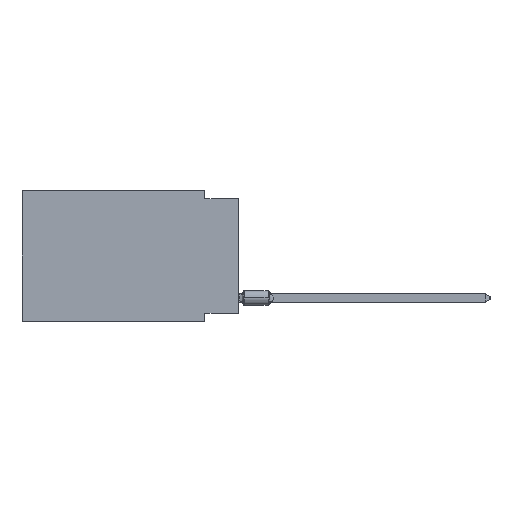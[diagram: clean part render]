
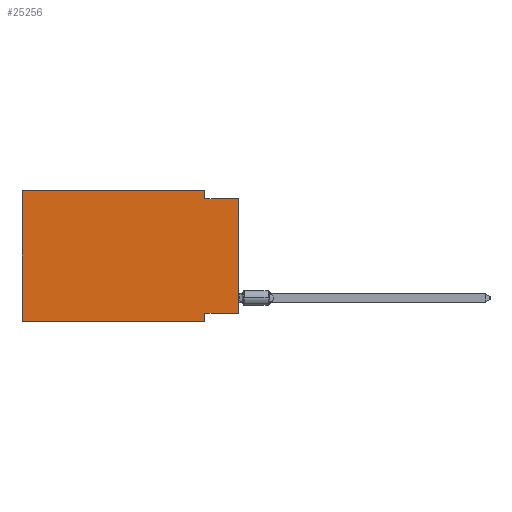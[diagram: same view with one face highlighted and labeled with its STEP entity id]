
A CAD part, left-side view. The second image highlights one B-rep face of the part: STEP entity #25256.
In plain terms, the highlighted planar face has unit normal (-1, 0, 0).
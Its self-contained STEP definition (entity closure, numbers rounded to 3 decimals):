
#961 = CARTESIAN_POINT ( 'NONE',  ( 0., 2.54, -9.271 ) ) ;
#1112 = ORIENTED_EDGE ( 'NONE', *, *, #34179, .T. ) ;
#2517 = DIRECTION ( 'NONE',  ( 0., 0., 1. ) ) ;
#2837 = PLANE ( 'NONE',  #8391 ) ;
#3027 = DIRECTION ( 'NONE',  ( 0., 0., -1. ) ) ;
#3663 = CARTESIAN_POINT ( 'NONE',  ( 0., 16.383, -9.906 ) ) ;
#4486 = CARTESIAN_POINT ( 'NONE',  ( 0., 16.383, 0. ) ) ;
#4726 = CARTESIAN_POINT ( 'NONE',  ( 0., 2.54, -9.906 ) ) ;
#4928 = CARTESIAN_POINT ( 'NONE',  ( 0., 2.54, 0. ) ) ;
#5298 = ORIENTED_EDGE ( 'NONE', *, *, #18529, .T. ) ;
#6240 = VERTEX_POINT ( 'NONE', #35952 ) ;
#6305 = CARTESIAN_POINT ( 'NONE',  ( 0., 16.383, 0. ) ) ;
#6789 = CARTESIAN_POINT ( 'NONE',  ( 0., 16.383, 0. ) ) ;
#7111 = VERTEX_POINT ( 'NONE', #961 ) ;
#7536 = VERTEX_POINT ( 'NONE', #6789 ) ;
#7638 = VECTOR ( 'NONE', #27860, 1000. ) ;
#7889 = EDGE_CURVE ( 'NONE', #31201, #7111, #28118, .T. ) ;
#8057 = LINE ( 'NONE', #35764, #11187 ) ;
#8391 = AXIS2_PLACEMENT_3D ( 'NONE', #11437, #14175, #3027 ) ;
#9229 = LINE ( 'NONE', #25482, #7638 ) ;
#9932 = VECTOR ( 'NONE', #11055, 1000. ) ;
#10415 = ORIENTED_EDGE ( 'NONE', *, *, #7889, .F. ) ;
#10790 = EDGE_LOOP ( 'NONE', ( #5298, #18662, #32331, #12112, #18404, #1112, #22360, #10415 ) ) ;
#10972 = DIRECTION ( 'NONE',  ( 0., 1., 0. ) ) ;
#11055 = DIRECTION ( 'NONE',  ( 0., -1., 0. ) ) ;
#11187 = VECTOR ( 'NONE', #16255, 1000. ) ;
#11437 = CARTESIAN_POINT ( 'NONE',  ( 0., 16.383, 0. ) ) ;
#12112 = ORIENTED_EDGE ( 'NONE', *, *, #26755, .F. ) ;
#12121 = VECTOR ( 'NONE', #26473, 1000. ) ;
#13576 = VERTEX_POINT ( 'NONE', #4726 ) ;
#14175 = DIRECTION ( 'NONE',  ( 1., 0., 0. ) ) ;
#14190 = CARTESIAN_POINT ( 'NONE',  ( 0., 16.383, -9.906 ) ) ;
#14340 = VECTOR ( 'NONE', #23251, 1000. ) ;
#14860 = LINE ( 'NONE', #31459, #14340 ) ;
#15666 = EDGE_CURVE ( 'NONE', #23734, #6240, #24730, .T. ) ;
#15969 = LINE ( 'NONE', #4486, #35739 ) ;
#16255 = DIRECTION ( 'NONE',  ( 0., 0., -1. ) ) ;
#16623 = CARTESIAN_POINT ( 'NONE',  ( 0., 0., -9.271 ) ) ;
#18404 = ORIENTED_EDGE ( 'NONE', *, *, #29255, .F. ) ;
#18529 = EDGE_CURVE ( 'NONE', #31201, #6240, #14860, .T. ) ;
#18662 = ORIENTED_EDGE ( 'NONE', *, *, #15666, .F. ) ;
#19645 = FACE_OUTER_BOUND ( 'NONE', #10790, .T. ) ;
#20950 = EDGE_CURVE ( 'NONE', #7111, #13576, #8057, .T. ) ;
#21760 = VERTEX_POINT ( 'NONE', #14190 ) ;
#21780 = EDGE_CURVE ( 'NONE', #28673, #23734, #9229, .T. ) ;
#22360 = ORIENTED_EDGE ( 'NONE', *, *, #20950, .F. ) ;
#22501 = CARTESIAN_POINT ( 'NONE',  ( 0., 0., -9.271 ) ) ;
#23251 = DIRECTION ( 'NONE',  ( 0., 0., 1. ) ) ;
#23734 = VERTEX_POINT ( 'NONE', #34700 ) ;
#24730 = LINE ( 'NONE', #27096, #9932 ) ;
#25256 = ADVANCED_FACE ( 'NONE', ( #19645 ), #2837, .F. ) ;
#25482 = CARTESIAN_POINT ( 'NONE',  ( 0., 2.54, 0. ) ) ;
#26473 = DIRECTION ( 'NONE',  ( 0., -1., 0. ) ) ;
#26745 = DIRECTION ( 'NONE',  ( 0., -1., 0. ) ) ;
#26755 = EDGE_CURVE ( 'NONE', #7536, #28673, #15969, .T. ) ;
#27096 = CARTESIAN_POINT ( 'NONE',  ( 0., 0., -0.635 ) ) ;
#27860 = DIRECTION ( 'NONE',  ( 0., 0., -1. ) ) ;
#28118 = LINE ( 'NONE', #16623, #33492 ) ;
#28673 = VERTEX_POINT ( 'NONE', #4928 ) ;
#29255 = EDGE_CURVE ( 'NONE', #21760, #7536, #31309, .T. ) ;
#31201 = VERTEX_POINT ( 'NONE', #22501 ) ;
#31309 = LINE ( 'NONE', #6305, #35275 ) ;
#31459 = CARTESIAN_POINT ( 'NONE',  ( 0., 0., 0. ) ) ;
#32331 = ORIENTED_EDGE ( 'NONE', *, *, #21780, .F. ) ;
#33492 = VECTOR ( 'NONE', #10972, 1000. ) ;
#34179 = EDGE_CURVE ( 'NONE', #21760, #13576, #34308, .T. ) ;
#34308 = LINE ( 'NONE', #3663, #12121 ) ;
#34700 = CARTESIAN_POINT ( 'NONE',  ( 0., 2.54, -0.635 ) ) ;
#35275 = VECTOR ( 'NONE', #2517, 1000. ) ;
#35739 = VECTOR ( 'NONE', #26745, 1000. ) ;
#35764 = CARTESIAN_POINT ( 'NONE',  ( 0., 2.54, -9.906 ) ) ;
#35952 = CARTESIAN_POINT ( 'NONE',  ( 0., 0., -0.635 ) ) ;
